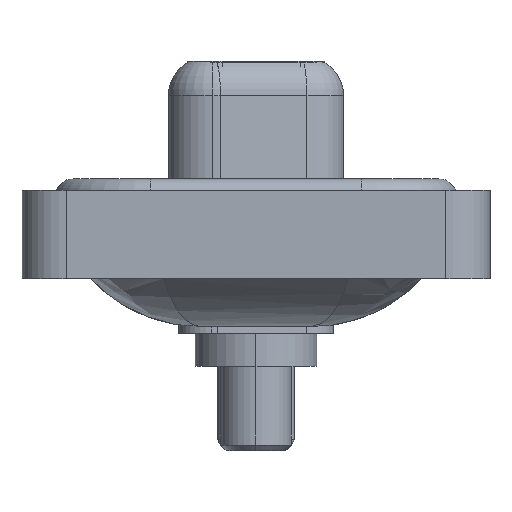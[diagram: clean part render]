
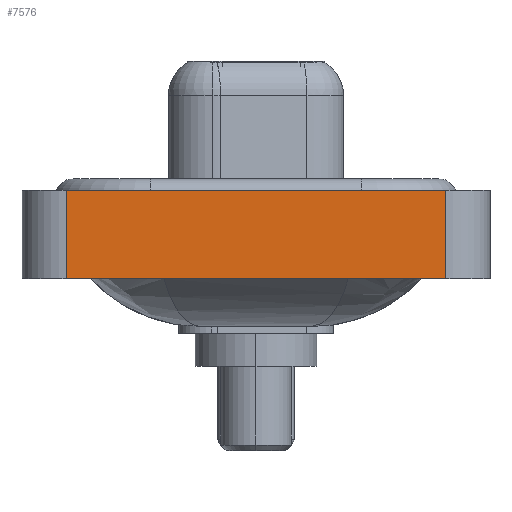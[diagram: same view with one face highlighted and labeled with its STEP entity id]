
A CAD part, left-side view. The second image highlights one B-rep face of the part: STEP entity #7576.
In plain terms, the highlighted planar face has unit normal (-1, 0, 0).
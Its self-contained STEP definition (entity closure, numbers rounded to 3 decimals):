
#269 = LINE ( 'NONE', #20029, #8181 ) ;
#796 = CARTESIAN_POINT ( 'NONE',  ( -7.35, -8.55, 0.4 ) ) ;
#1321 = EDGE_LOOP ( 'NONE', ( #8301, #18482, #6457, #13923 ) ) ;
#2107 = DIRECTION ( 'NONE',  ( 0., 0., 1. ) ) ;
#2899 = EDGE_CURVE ( 'NONE', #7647, #14128, #14953, .T. ) ;
#3406 = CARTESIAN_POINT ( 'NONE',  ( -7.35, -8.55, -3.6 ) ) ;
#4698 = EDGE_CURVE ( 'NONE', #7647, #17190, #269, .T. ) ;
#4922 = VERTEX_POINT ( 'NONE', #9101 ) ;
#6151 = EDGE_CURVE ( 'NONE', #14128, #4922, #9103, .T. ) ;
#6457 = ORIENTED_EDGE ( 'NONE', *, *, #2899, .F. ) ;
#7036 = DIRECTION ( 'NONE',  ( 0., 0., 1. ) ) ;
#7576 = ADVANCED_FACE ( 'NONE', ( #11574 ), #17960, .T. ) ;
#7647 = VERTEX_POINT ( 'NONE', #11466 ) ;
#8181 = VECTOR ( 'NONE', #11629, 1000. ) ;
#8301 = ORIENTED_EDGE ( 'NONE', *, *, #16286, .T. ) ;
#8609 = CARTESIAN_POINT ( 'NONE',  ( -7.35, 8.55, -3.6 ) ) ;
#8670 = AXIS2_PLACEMENT_3D ( 'NONE', #3406, #19550, #7036 ) ;
#9101 = CARTESIAN_POINT ( 'NONE',  ( -7.35, -8.55, 0.4 ) ) ;
#9103 = LINE ( 'NONE', #796, #13324 ) ;
#9367 = VECTOR ( 'NONE', #2107, 1000. ) ;
#11287 = CARTESIAN_POINT ( 'NONE',  ( -7.35, 8.55, 0.4 ) ) ;
#11466 = CARTESIAN_POINT ( 'NONE',  ( -7.35, 8.55, -3.6 ) ) ;
#11574 = FACE_OUTER_BOUND ( 'NONE', #1321, .T. ) ;
#11629 = DIRECTION ( 'NONE',  ( 0., -1., 0. ) ) ;
#13053 = CARTESIAN_POINT ( 'NONE',  ( -7.35, -8.55, -3.6 ) ) ;
#13144 = DIRECTION ( 'NONE',  ( 0., 0., 1. ) ) ;
#13324 = VECTOR ( 'NONE', #17167, 1000. ) ;
#13638 = VECTOR ( 'NONE', #13144, 1000. ) ;
#13923 = ORIENTED_EDGE ( 'NONE', *, *, #4698, .T. ) ;
#14128 = VERTEX_POINT ( 'NONE', #11287 ) ;
#14850 = LINE ( 'NONE', #18147, #9367 ) ;
#14953 = LINE ( 'NONE', #8609, #13638 ) ;
#16286 = EDGE_CURVE ( 'NONE', #17190, #4922, #14850, .T. ) ;
#17167 = DIRECTION ( 'NONE',  ( 0., -1., 0. ) ) ;
#17190 = VERTEX_POINT ( 'NONE', #13053 ) ;
#17960 = PLANE ( 'NONE',  #8670 ) ;
#18147 = CARTESIAN_POINT ( 'NONE',  ( -7.35, -8.55, -3.6 ) ) ;
#18482 = ORIENTED_EDGE ( 'NONE', *, *, #6151, .F. ) ;
#19550 = DIRECTION ( 'NONE',  ( -1., 0., 0. ) ) ;
#20029 = CARTESIAN_POINT ( 'NONE',  ( -7.35, -8.55, -3.6 ) ) ;
